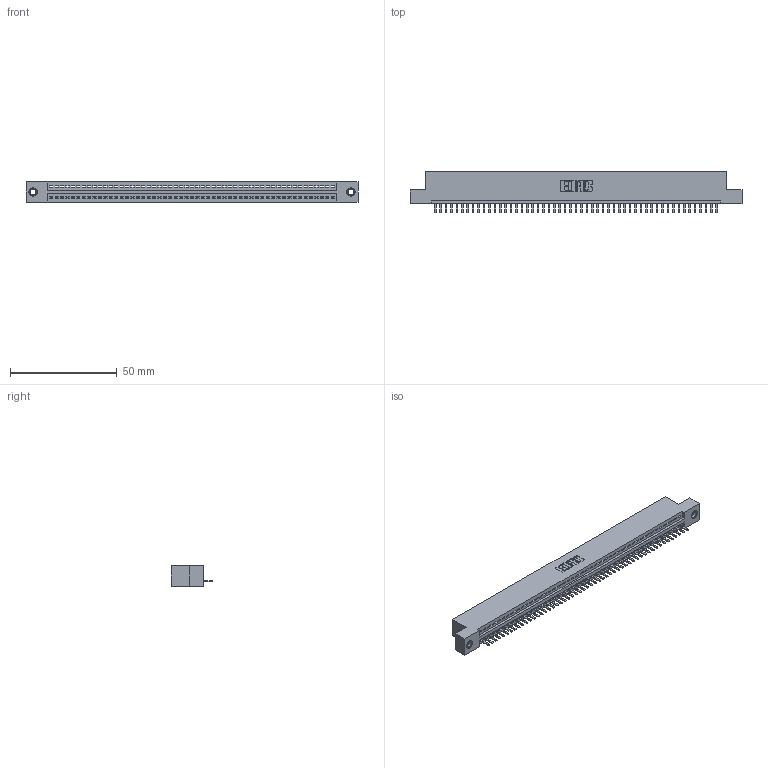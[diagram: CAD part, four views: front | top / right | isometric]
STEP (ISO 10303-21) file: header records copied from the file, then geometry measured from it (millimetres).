
FILE_DESCRIPTION (( 'STEP AP203' ), '1' );
FILE_NAME ('395-053-520-107.STEP', '2019-10-23T13:47:38', ( '' ), ( '' ), 'SwSTEP 2.0', 'SolidWorks 2016', '' );
FILE_SCHEMA (( 'CONFIG_CONTROL_DESIGN' ));
Length unit declared in the file: inch
Products named in the file (4): 345-292-001_345-293-120; 395-053-520-107; 345 Part_Flush Mounting Lugs - 0.156 Dia-TI; 345-250-001_345-250-005-103
Assembly tree (56 placements, depth 2):
  395-053-520-107
    345 Part_Flush Mounting Lugs - 0.156 Dia-TI
    345-292-001_345-293-120  x53
    345-250-001_345-250-005-103  x2
Bounding box: 155.83 x 19.68 x 9.4 mm (x, y, z)
Volume: 14724.9 mm3; surface area: 19251.4 mm2
Topology: 56 solids, 56 shells, 3472 faces, 10229 edges, 6670 vertices
Faces by surface type: plane 2338, cylinder 1118, cone 12, torus 4
Entity records: 39708 total; most frequent: CARTESIAN_POINT 6870, ORIENTED_EDGE 6838, DIRECTION 5999, EDGE_CURVE 3419, LINE 3051, VECTOR 3051, VERTEX_POINT 2272, AXIS2_PLACEMENT_3D 1474
